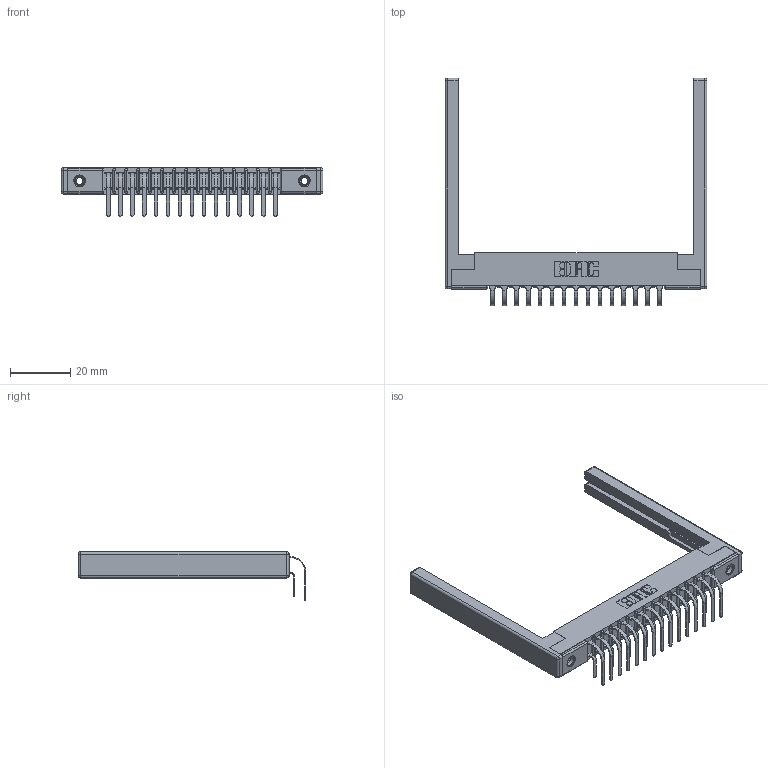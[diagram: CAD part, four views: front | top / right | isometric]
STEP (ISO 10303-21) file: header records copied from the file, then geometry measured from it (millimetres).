
FILE_DESCRIPTION (( 'STEP AP203' ), '1' );
FILE_NAME ('307-030-559-268.STEP', '2022-07-08T15:58:58', ( '' ), ( '' ), 'SwSTEP 2.0', 'SolidWorks 2020', '' );
FILE_SCHEMA (( 'CONFIG_CONTROL_DESIGN' ));
Length unit declared in the file: inch
Products named in the file (6): 307 Part_.156 Dia Mounting Holes; 307-290-001_558 559 - 1 (Single); 307-220-068; 307-290-001_559 - 2 (Single); 345-250-001_345-250-001-102; 307-030-559-268
Assembly tree (35 placements, depth 2):
  307-030-559-268
    307 Part_.156 Dia Mounting Holes
    307-290-001_558 559 - 1 (Single)  x15
    307-290-001_559 - 2 (Single)  x15
    307-220-068  x2
    345-250-001_345-250-001-102  x2
Bounding box: 86.87 x 75.48 x 16.08 mm (x, y, z)
Volume: 10357.2 mm3; surface area: 14543.2 mm2
Topology: 35 solids, 35 shells, 1788 faces, 4973 edges, 3210 vertices
Faces by surface type: plane 1148, cylinder 584, sphere 40, cone 12, torus 4
Entity records: 20874 total; most frequent: CARTESIAN_POINT 3402, ORIENTED_EDGE 3360, DIRECTION 3358, EDGE_CURVE 1680, LINE 1274, VECTOR 1274, VERTEX_POINT 1086, AXIS2_PLACEMENT_3D 1042
